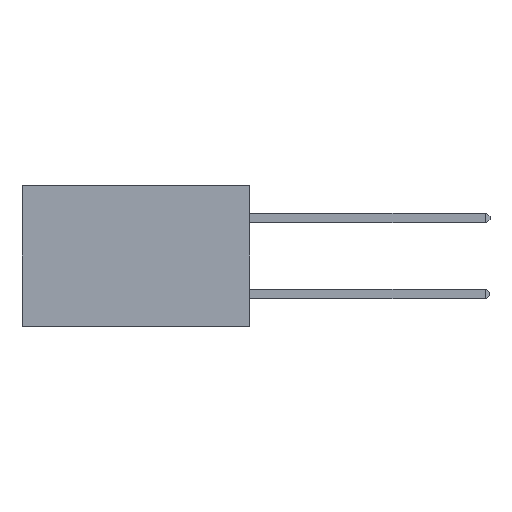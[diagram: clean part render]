
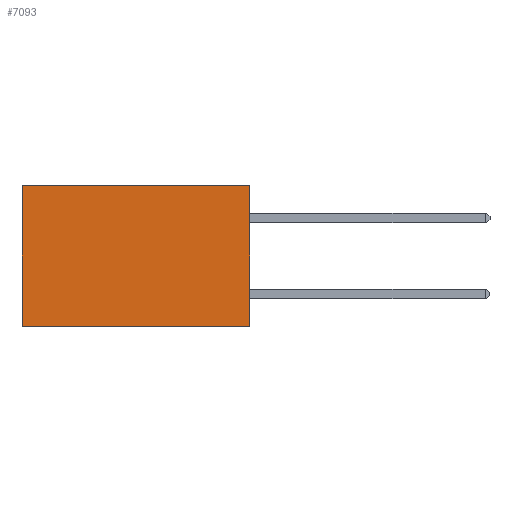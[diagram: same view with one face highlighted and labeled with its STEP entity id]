
A CAD part, left-side view. The second image highlights one B-rep face of the part: STEP entity #7093.
In plain terms, the highlighted planar face has unit normal (-1, 0, 0).
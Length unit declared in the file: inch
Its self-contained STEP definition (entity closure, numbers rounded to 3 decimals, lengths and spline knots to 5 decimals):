
#1526 = VERTEX_POINT ( 'NONE', #2497 ) ;
#2497 = CARTESIAN_POINT ( 'NONE',  ( 0.2875, 0.6, 0. ) ) ;
#2695 = LINE ( 'NONE', #8756, #17330 ) ;
#2723 = EDGE_CURVE ( 'NONE', #17738, #17655, #10597, .T. ) ;
#2940 = VECTOR ( 'NONE', #14446, 39.37008 ) ;
#3583 = DIRECTION ( 'NONE',  ( 0., 0., -1. ) ) ;
#4692 = ORIENTED_EDGE ( 'NONE', *, *, #10088, .T. ) ;
#4917 = PLANE ( 'NONE',  #17123 ) ;
#5759 = EDGE_LOOP ( 'NONE', ( #16366, #15824, #18176, #4692 ) ) ;
#6049 = VECTOR ( 'NONE', #3583, 39.37008 ) ;
#6392 = DIRECTION ( 'NONE',  ( 1., 0., 0. ) ) ;
#6558 = VECTOR ( 'NONE', #9178, 39.37008 ) ;
#7093 = ADVANCED_FACE ( 'NONE', ( #8302 ), #4917, .F. ) ;
#8302 = FACE_OUTER_BOUND ( 'NONE', #5759, .T. ) ;
#8406 = CARTESIAN_POINT ( 'NONE',  ( 0.2875, 0.6, -0.37 ) ) ;
#8756 = CARTESIAN_POINT ( 'NONE',  ( 0.2875, 0., 0. ) ) ;
#9178 = DIRECTION ( 'NONE',  ( 0., 1., 0. ) ) ;
#10088 = EDGE_CURVE ( 'NONE', #17738, #1526, #2695, .T. ) ;
#10597 = LINE ( 'NONE', #14643, #2940 ) ;
#10895 = CARTESIAN_POINT ( 'NONE',  ( 0.2875, 0., -0.37 ) ) ;
#11542 = DIRECTION ( 'NONE',  ( 0., 1., 0. ) ) ;
#13088 = LINE ( 'NONE', #16232, #6049 ) ;
#13158 = EDGE_CURVE ( 'NONE', #17655, #17211, #14464, .T. ) ;
#13331 = CARTESIAN_POINT ( 'NONE',  ( 0.2875, 0., 0. ) ) ;
#13359 = CARTESIAN_POINT ( 'NONE',  ( 0.2875, 0., -0.37 ) ) ;
#13871 = CARTESIAN_POINT ( 'NONE',  ( 0.2875, 0., 0. ) ) ;
#14446 = DIRECTION ( 'NONE',  ( 0., 0., -1. ) ) ;
#14464 = LINE ( 'NONE', #13359, #6558 ) ;
#14643 = CARTESIAN_POINT ( 'NONE',  ( 0.2875, 0., 0. ) ) ;
#15824 = ORIENTED_EDGE ( 'NONE', *, *, #13158, .F. ) ;
#16225 = DIRECTION ( 'NONE',  ( 0., 0., -1. ) ) ;
#16232 = CARTESIAN_POINT ( 'NONE',  ( 0.2875, 0.6, 0. ) ) ;
#16366 = ORIENTED_EDGE ( 'NONE', *, *, #17000, .T. ) ;
#17000 = EDGE_CURVE ( 'NONE', #1526, #17211, #13088, .T. ) ;
#17123 = AXIS2_PLACEMENT_3D ( 'NONE', #13331, #6392, #16225 ) ;
#17211 = VERTEX_POINT ( 'NONE', #8406 ) ;
#17330 = VECTOR ( 'NONE', #11542, 39.37008 ) ;
#17655 = VERTEX_POINT ( 'NONE', #10895 ) ;
#17738 = VERTEX_POINT ( 'NONE', #13871 ) ;
#18176 = ORIENTED_EDGE ( 'NONE', *, *, #2723, .F. ) ;
